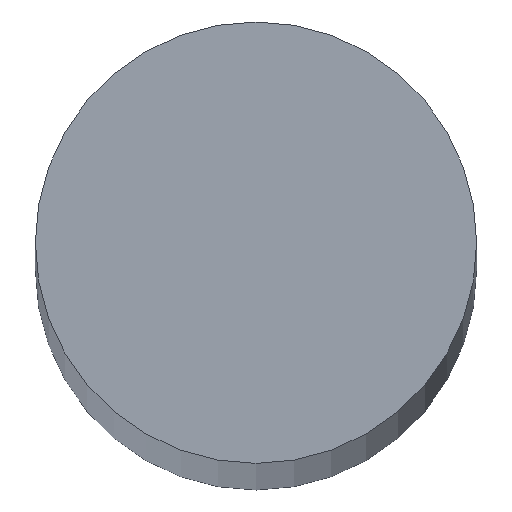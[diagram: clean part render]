
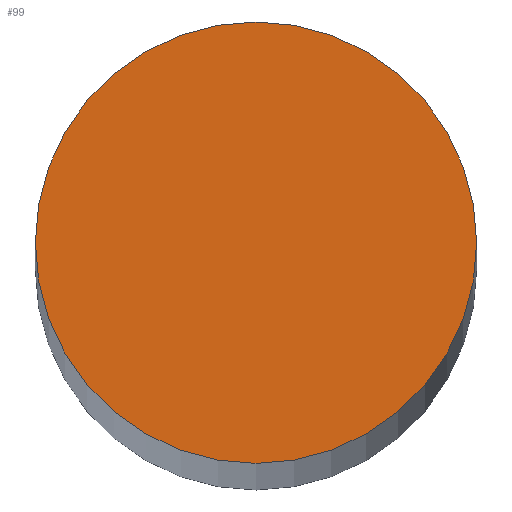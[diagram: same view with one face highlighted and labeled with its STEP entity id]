
A CAD part, top view. The second image highlights one B-rep face of the part: STEP entity #99.
In plain terms, the highlighted planar face has unit normal (0, 0, 1).
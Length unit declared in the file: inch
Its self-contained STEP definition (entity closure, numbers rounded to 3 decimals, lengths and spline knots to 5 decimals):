
#1 = CIRCLE ( 'NONE', #132, 0.09843 ) ;
#8 = DIRECTION ( 'NONE',  ( -1., 0., 0. ) ) ;
#11 = CARTESIAN_POINT ( 'NONE',  ( 0., 0., 6. ) ) ;
#13 = ORIENTED_EDGE ( 'NONE', *, *, #19, .T. ) ;
#14 = ORIENTED_EDGE ( 'NONE', *, *, #61, .T. ) ;
#19 = EDGE_CURVE ( 'NONE', #48, #141, #35, .T. ) ;
#21 = CARTESIAN_POINT ( 'NONE',  ( -0.09843, 0., 6. ) ) ;
#28 = DIRECTION ( 'NONE',  ( 0., 0., 1. ) ) ;
#29 = FACE_OUTER_BOUND ( 'NONE', #131, .T. ) ;
#35 = CIRCLE ( 'NONE', #125, 0.09843 ) ;
#47 = DIRECTION ( 'NONE',  ( 0., 0., 1. ) ) ;
#48 = VERTEX_POINT ( 'NONE', #124 ) ;
#61 = EDGE_CURVE ( 'NONE', #141, #48, #1, .T. ) ;
#71 = PLANE ( 'NONE',  #130 ) ;
#78 = DIRECTION ( 'NONE',  ( -1., 0., 0. ) ) ;
#87 = DIRECTION ( 'NONE',  ( 0., 0., 1. ) ) ;
#97 = DIRECTION ( 'NONE',  ( 1., 0., 0. ) ) ;
#98 = CARTESIAN_POINT ( 'NONE',  ( 0., 0., 6. ) ) ;
#99 = ADVANCED_FACE ( 'NONE', ( #29 ), #71, .T. ) ;
#124 = CARTESIAN_POINT ( 'NONE',  ( 0.09843, 0., 6. ) ) ;
#125 = AXIS2_PLACEMENT_3D ( 'NONE', #98, #87, #8 ) ;
#129 = CARTESIAN_POINT ( 'NONE',  ( 0., 0., 6. ) ) ;
#130 = AXIS2_PLACEMENT_3D ( 'NONE', #11, #28, #97 ) ;
#131 = EDGE_LOOP ( 'NONE', ( #13, #14 ) ) ;
#132 = AXIS2_PLACEMENT_3D ( 'NONE', #129, #47, #78 ) ;
#141 = VERTEX_POINT ( 'NONE', #21 ) ;
